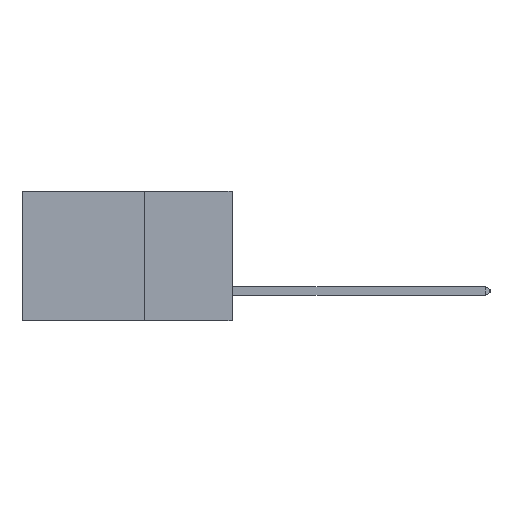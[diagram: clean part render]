
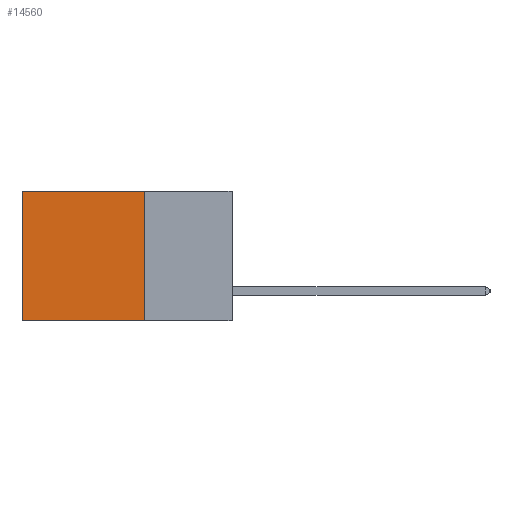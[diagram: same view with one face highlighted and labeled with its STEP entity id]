
A CAD part, left-side view. The second image highlights one B-rep face of the part: STEP entity #14560.
In plain terms, the highlighted planar face has unit normal (-1, 0, 0).
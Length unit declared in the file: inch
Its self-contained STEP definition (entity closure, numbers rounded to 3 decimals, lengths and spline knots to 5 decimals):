
#69 = VERTEX_POINT ( 'NONE', #11054 ) ;
#1302 = VERTEX_POINT ( 'NONE', #2428 ) ;
#1328 = CARTESIAN_POINT ( 'NONE',  ( 0.2875, 0.25, 0. ) ) ;
#1510 = EDGE_CURVE ( 'NONE', #69, #11404, #3028, .T. ) ;
#1876 = ORIENTED_EDGE ( 'NONE', *, *, #4518, .T. ) ;
#2409 = CARTESIAN_POINT ( 'NONE',  ( 0.2875, 0.25, -0.37 ) ) ;
#2428 = CARTESIAN_POINT ( 'NONE',  ( 0.2875, 0.25, 0. ) ) ;
#3028 = LINE ( 'NONE', #2409, #16426 ) ;
#3148 = DIRECTION ( 'NONE',  ( 0., 0., -1. ) ) ;
#3481 = EDGE_LOOP ( 'NONE', ( #1876, #13953, #7330, #3802 ) ) ;
#3802 = ORIENTED_EDGE ( 'NONE', *, *, #15025, .T. ) ;
#4518 = EDGE_CURVE ( 'NONE', #13236, #11404, #14384, .T. ) ;
#4915 = CARTESIAN_POINT ( 'NONE',  ( 0.2875, 0.25, 0. ) ) ;
#4941 = CARTESIAN_POINT ( 'NONE',  ( 0.2875, 0.25, 0. ) ) ;
#5216 = PLANE ( 'NONE',  #9756 ) ;
#5427 = FACE_OUTER_BOUND ( 'NONE', #3481, .T. ) ;
#5791 = DIRECTION ( 'NONE',  ( 0., 1., 0. ) ) ;
#6536 = DIRECTION ( 'NONE',  ( 0., 0., -1. ) ) ;
#7131 = EDGE_CURVE ( 'NONE', #1302, #69, #16516, .T. ) ;
#7330 = ORIENTED_EDGE ( 'NONE', *, *, #7131, .F. ) ;
#7503 = VECTOR ( 'NONE', #3148, 39.37008 ) ;
#9756 = AXIS2_PLACEMENT_3D ( 'NONE', #1328, #14274, #6536 ) ;
#10712 = CARTESIAN_POINT ( 'NONE',  ( 0.2875, 0.6, 0. ) ) ;
#10986 = CARTESIAN_POINT ( 'NONE',  ( 0.2875, 0.6, -0.37 ) ) ;
#11054 = CARTESIAN_POINT ( 'NONE',  ( 0.2875, 0.25, -0.37 ) ) ;
#11390 = DIRECTION ( 'NONE',  ( 0., 0., -1. ) ) ;
#11404 = VERTEX_POINT ( 'NONE', #10986 ) ;
#11480 = VECTOR ( 'NONE', #12683, 39.37008 ) ;
#12683 = DIRECTION ( 'NONE',  ( 0., 1., 0. ) ) ;
#13062 = VECTOR ( 'NONE', #11390, 39.37008 ) ;
#13236 = VERTEX_POINT ( 'NONE', #10712 ) ;
#13953 = ORIENTED_EDGE ( 'NONE', *, *, #1510, .F. ) ;
#14274 = DIRECTION ( 'NONE',  ( 1., 0., 0. ) ) ;
#14384 = LINE ( 'NONE', #14836, #7503 ) ;
#14560 = ADVANCED_FACE ( 'NONE', ( #5427 ), #5216, .F. ) ;
#14836 = CARTESIAN_POINT ( 'NONE',  ( 0.2875, 0.6, 0. ) ) ;
#14933 = LINE ( 'NONE', #4915, #11480 ) ;
#15025 = EDGE_CURVE ( 'NONE', #1302, #13236, #14933, .T. ) ;
#16426 = VECTOR ( 'NONE', #5791, 39.37008 ) ;
#16516 = LINE ( 'NONE', #4941, #13062 ) ;
